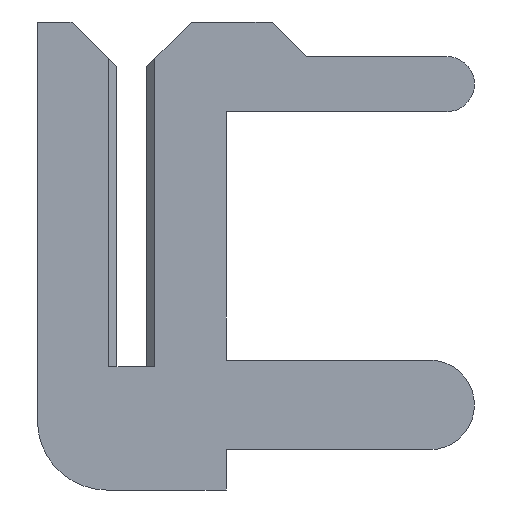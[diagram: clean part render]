
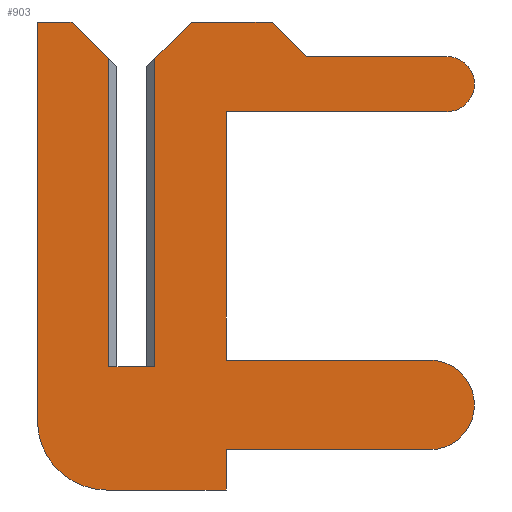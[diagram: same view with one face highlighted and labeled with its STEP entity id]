
A CAD part, left-side view. The second image highlights one B-rep face of the part: STEP entity #903.
In plain terms, the highlighted planar face has unit normal (-1, 0, 0).
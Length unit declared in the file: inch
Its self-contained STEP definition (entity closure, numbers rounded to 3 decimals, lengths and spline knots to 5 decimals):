
#18 = DIRECTION ( 'NONE',  ( 1., 0., 0. ) ) ;
#20 = ORIENTED_EDGE ( 'NONE', *, *, #310, .F. ) ;
#34 = CARTESIAN_POINT ( 'NONE',  ( -0.01, -0.01, 0. ) ) ;
#40 = DIRECTION ( 'NONE',  ( 0., -1., 0. ) ) ;
#46 = CARTESIAN_POINT ( 'NONE',  ( -0.01, 0.0065, 0.1305 ) ) ;
#50 = CIRCLE ( 'NONE', #1264, 0.0195 ) ;
#54 = CARTESIAN_POINT ( 'NONE',  ( -0.01, -0.1295, 0.003 ) ) ;
#63 = DIRECTION ( 'NONE',  ( 1., 0., 0. ) ) ;
#65 = ORIENTED_EDGE ( 'NONE', *, *, #385, .F. ) ;
#68 = LINE ( 'NONE', #1531, #400 ) ;
#90 = DIRECTION ( 'NONE',  ( 0., 0., 1. ) ) ;
#100 = LINE ( 'NONE', #1437, #1460 ) ;
#102 = DIRECTION ( 'NONE',  ( -1., 0., 0. ) ) ;
#108 = CARTESIAN_POINT ( 'NONE',  ( -0.01, -0.01, 0.15 ) ) ;
#116 = LINE ( 'NONE', #1648, #587 ) ;
#119 = EDGE_CURVE ( 'NONE', #751, #168, #161, .T. ) ;
#142 = ORIENTED_EDGE ( 'NONE', *, *, #1342, .F. ) ;
#144 = DIRECTION ( 'NONE',  ( 0., -1., 0. ) ) ;
#151 = DIRECTION ( 'NONE',  ( 0., 1., 0. ) ) ;
#161 = LINE ( 'NONE', #163, #275 ) ;
#163 = CARTESIAN_POINT ( 'NONE',  ( -0.01, -0.041, 0.003 ) ) ;
#168 = VERTEX_POINT ( 'NONE', #1359 ) ;
#171 = CARTESIAN_POINT ( 'NONE',  ( -0.01, -0.076, 0.135 ) ) ;
#186 = VECTOR ( 'NONE', #151, 39.37008 ) ;
#190 = ORIENTED_EDGE ( 'NONE', *, *, #600, .F. ) ;
#202 = EDGE_CURVE ( 'NONE', #232, #684, #116, .T. ) ;
#210 = LINE ( 'NONE', #171, #793 ) ;
#225 = EDGE_CURVE ( 'NONE', #646, #615, #210, .T. ) ;
#232 = VERTEX_POINT ( 'NONE', #857 ) ;
#237 = CARTESIAN_POINT ( 'NONE',  ( -0.01, -0.041, -0.0535 ) ) ;
#243 = LINE ( 'NONE', #108, #873 ) ;
#273 = CARTESIAN_POINT ( 'NONE',  ( -0.01, -0.041, -0.036 ) ) ;
#275 = VECTOR ( 'NONE', #322, 39.37008 ) ;
#282 = DIRECTION ( 'NONE',  ( 0., -1., 0. ) ) ;
#285 = AXIS2_PLACEMENT_3D ( 'NONE', #313, #295, #1224 ) ;
#289 = DIRECTION ( 'NONE',  ( 0., -1., 0. ) ) ;
#293 = CIRCLE ( 'NONE', #285, 0.012 ) ;
#295 = DIRECTION ( 'NONE',  ( 1., 0., 0. ) ) ;
#310 = EDGE_CURVE ( 'NONE', #804, #646, #1566, .T. ) ;
#313 = CARTESIAN_POINT ( 'NONE',  ( -0.01, -0.137, 0.123 ) ) ;
#322 = DIRECTION ( 'NONE',  ( 0., 0., -1. ) ) ;
#362 = ORIENTED_EDGE ( 'NONE', *, *, #409, .F. ) ;
#365 = EDGE_CURVE ( 'NONE', #1609, #751, #909, .T. ) ;
#378 = PLANE ( 'NONE',  #763 ) ;
#382 = VERTEX_POINT ( 'NONE', #826 ) ;
#385 = EDGE_CURVE ( 'NONE', #950, #1593, #1049, .T. ) ;
#394 = EDGE_CURVE ( 'NONE', #168, #704, #477, .T. ) ;
#400 = VECTOR ( 'NONE', #40, 39.37008 ) ;
#402 = EDGE_CURVE ( 'NONE', #864, #910, #649, .T. ) ;
#409 = EDGE_CURVE ( 'NONE', #1329, #1609, #293, .T. ) ;
#442 = CARTESIAN_POINT ( 'NONE',  ( -0.01, 0.011, -0.0235 ) ) ;
#447 = EDGE_LOOP ( 'NONE', ( #1201, #844, #142, #567, #190, #1583, #656, #65, #746, #1372, #1441, #817, #918, #871, #635, #362, #1209, #1106, #20 ) ) ;
#470 = EDGE_CURVE ( 'NONE', #615, #1329, #68, .T. ) ;
#477 = LINE ( 'NONE', #1346, #1645 ) ;
#515 = CARTESIAN_POINT ( 'NONE',  ( -0.01, -0.137, 0.135 ) ) ;
#527 = CARTESIAN_POINT ( 'NONE',  ( -0.01, 0.011, -0.0535 ) ) ;
#546 = VERTEX_POINT ( 'NONE', #34 ) ;
#560 = VECTOR ( 'NONE', #982, 39.37008 ) ;
#567 = ORIENTED_EDGE ( 'NONE', *, *, #202, .T. ) ;
#571 = CARTESIAN_POINT ( 'NONE',  ( -0.01, 0.026, 0.15 ) ) ;
#587 = VECTOR ( 'NONE', #850, 39.37008 ) ;
#600 = EDGE_CURVE ( 'NONE', #910, #684, #1675, .T. ) ;
#615 = VERTEX_POINT ( 'NONE', #1008 ) ;
#635 = ORIENTED_EDGE ( 'NONE', *, *, #365, .F. ) ;
#646 = VERTEX_POINT ( 'NONE', #1131 ) ;
#649 = LINE ( 'NONE', #571, #560 ) ;
#656 = ORIENTED_EDGE ( 'NONE', *, *, #707, .F. ) ;
#669 = AXIS2_PLACEMENT_3D ( 'NONE', #442, #18, #1483 ) ;
#684 = VERTEX_POINT ( 'NONE', #1391 ) ;
#686 = EDGE_CURVE ( 'NONE', #382, #950, #1277, .T. ) ;
#701 = CARTESIAN_POINT ( 'NONE',  ( -0.01, -0.137, 0.111 ) ) ;
#704 = VERTEX_POINT ( 'NONE', #54 ) ;
#707 = EDGE_CURVE ( 'NONE', #1593, #864, #1629, .T. ) ;
#718 = VECTOR ( 'NONE', #282, 39.37008 ) ;
#719 = DIRECTION ( 'NONE',  ( 0., -0.707, -0.707 ) ) ;
#733 = DIRECTION ( 'NONE',  ( 0., 1., 0. ) ) ;
#745 = CARTESIAN_POINT ( 'NONE',  ( -0.01, 0.041, 0.15 ) ) ;
#746 = ORIENTED_EDGE ( 'NONE', *, *, #686, .F. ) ;
#751 = VERTEX_POINT ( 'NONE', #1293 ) ;
#763 = AXIS2_PLACEMENT_3D ( 'NONE', #1172, #102, #1601 ) ;
#765 = CARTESIAN_POINT ( 'NONE',  ( -0.01, 0.026, 0.15 ) ) ;
#784 = EDGE_CURVE ( 'NONE', #1418, #382, #1396, .T. ) ;
#793 = VECTOR ( 'NONE', #1341, 39.37008 ) ;
#796 = EDGE_CURVE ( 'NONE', #704, #1394, #50, .T. ) ;
#802 = CARTESIAN_POINT ( 'NONE',  ( -0.01, 0.0065, 0. ) ) ;
#803 = VECTOR ( 'NONE', #733, 39.37008 ) ;
#804 = VERTEX_POINT ( 'NONE', #1282 ) ;
#817 = ORIENTED_EDGE ( 'NONE', *, *, #796, .F. ) ;
#826 = CARTESIAN_POINT ( 'NONE',  ( -0.01, -0.041, -0.0535 ) ) ;
#844 = ORIENTED_EDGE ( 'NONE', *, *, #1058, .T. ) ;
#850 = DIRECTION ( 'NONE',  ( 0., 0., 1. ) ) ;
#857 = CARTESIAN_POINT ( 'NONE',  ( -0.01, 0.01, 0. ) ) ;
#864 = VERTEX_POINT ( 'NONE', #912 ) ;
#871 = ORIENTED_EDGE ( 'NONE', *, *, #119, .F. ) ;
#873 = VECTOR ( 'NONE', #1442, 39.37008 ) ;
#895 = VECTOR ( 'NONE', #719, 39.37008 ) ;
#903 = ADVANCED_FACE ( 'NONE', ( #1230 ), #378, .T. ) ;
#909 = LINE ( 'NONE', #1644, #186 ) ;
#910 = VERTEX_POINT ( 'NONE', #765 ) ;
#912 = CARTESIAN_POINT ( 'NONE',  ( -0.01, 0.041, 0.15 ) ) ;
#918 = ORIENTED_EDGE ( 'NONE', *, *, #394, .F. ) ;
#927 = LINE ( 'NONE', #802, #718 ) ;
#932 = CARTESIAN_POINT ( 'NONE',  ( -0.01, -0.01, 0.134 ) ) ;
#950 = VERTEX_POINT ( 'NONE', #527 ) ;
#958 = EDGE_CURVE ( 'NONE', #1394, #1418, #100, .T. ) ;
#982 = DIRECTION ( 'NONE',  ( 0., -1., 0. ) ) ;
#1008 = CARTESIAN_POINT ( 'NONE',  ( -0.01, -0.076, 0.135 ) ) ;
#1020 = DIRECTION ( 'NONE',  ( 0., 0., -1. ) ) ;
#1049 = CIRCLE ( 'NONE', #669, 0.03 ) ;
#1056 = VECTOR ( 'NONE', #1489, 39.37008 ) ;
#1058 = EDGE_CURVE ( 'NONE', #1316, #546, #243, .T. ) ;
#1096 = CARTESIAN_POINT ( 'NONE',  ( -0.01, 0.041, -0.0235 ) ) ;
#1106 = ORIENTED_EDGE ( 'NONE', *, *, #225, .F. ) ;
#1131 = CARTESIAN_POINT ( 'NONE',  ( -0.01, -0.061, 0.15 ) ) ;
#1172 = CARTESIAN_POINT ( 'NONE',  ( -0.01, 0.011, -0.0235 ) ) ;
#1201 = ORIENTED_EDGE ( 'NONE', *, *, #1323, .F. ) ;
#1205 = VECTOR ( 'NONE', #144, 39.37008 ) ;
#1209 = ORIENTED_EDGE ( 'NONE', *, *, #470, .F. ) ;
#1224 = DIRECTION ( 'NONE',  ( 0., 0., 1. ) ) ;
#1230 = FACE_OUTER_BOUND ( 'NONE', #447, .T. ) ;
#1264 = AXIS2_PLACEMENT_3D ( 'NONE', #1427, #63, #90 ) ;
#1277 = LINE ( 'NONE', #1665, #803 ) ;
#1282 = CARTESIAN_POINT ( 'NONE',  ( -0.01, -0.026, 0.15 ) ) ;
#1293 = CARTESIAN_POINT ( 'NONE',  ( -0.01, -0.041, 0.111 ) ) ;
#1312 = CARTESIAN_POINT ( 'NONE',  ( -0.01, -0.0065, 0.1305 ) ) ;
#1316 = VERTEX_POINT ( 'NONE', #932 ) ;
#1323 = EDGE_CURVE ( 'NONE', #1316, #804, #1696, .T. ) ;
#1329 = VERTEX_POINT ( 'NONE', #515 ) ;
#1341 = DIRECTION ( 'NONE',  ( 0., -0.707, -0.707 ) ) ;
#1342 = EDGE_CURVE ( 'NONE', #232, #546, #927, .T. ) ;
#1346 = CARTESIAN_POINT ( 'NONE',  ( -0.01, -0.1295, 0.003 ) ) ;
#1359 = CARTESIAN_POINT ( 'NONE',  ( -0.01, -0.041, 0.003 ) ) ;
#1363 = CARTESIAN_POINT ( 'NONE',  ( -0.01, -0.026, 0.15 ) ) ;
#1372 = ORIENTED_EDGE ( 'NONE', *, *, #784, .F. ) ;
#1391 = CARTESIAN_POINT ( 'NONE',  ( -0.01, 0.01, 0.134 ) ) ;
#1394 = VERTEX_POINT ( 'NONE', #1608 ) ;
#1396 = LINE ( 'NONE', #237, #1699 ) ;
#1418 = VERTEX_POINT ( 'NONE', #273 ) ;
#1427 = CARTESIAN_POINT ( 'NONE',  ( -0.01, -0.1295, -0.0165 ) ) ;
#1437 = CARTESIAN_POINT ( 'NONE',  ( -0.01, -0.041, -0.036 ) ) ;
#1441 = ORIENTED_EDGE ( 'NONE', *, *, #958, .F. ) ;
#1442 = DIRECTION ( 'NONE',  ( 0., 0., -1. ) ) ;
#1460 = VECTOR ( 'NONE', #1725, 39.37008 ) ;
#1483 = DIRECTION ( 'NONE',  ( 0., 0., 1. ) ) ;
#1489 = DIRECTION ( 'NONE',  ( 0., -0.707, 0.707 ) ) ;
#1531 = CARTESIAN_POINT ( 'NONE',  ( -0.01, -0.137, 0.135 ) ) ;
#1558 = DIRECTION ( 'NONE',  ( 0., 0., 1. ) ) ;
#1566 = LINE ( 'NONE', #1363, #1205 ) ;
#1583 = ORIENTED_EDGE ( 'NONE', *, *, #402, .F. ) ;
#1592 = VECTOR ( 'NONE', #1558, 39.37008 ) ;
#1593 = VERTEX_POINT ( 'NONE', #1096 ) ;
#1601 = DIRECTION ( 'NONE',  ( 0., 0., 1. ) ) ;
#1608 = CARTESIAN_POINT ( 'NONE',  ( -0.01, -0.1295, -0.036 ) ) ;
#1609 = VERTEX_POINT ( 'NONE', #701 ) ;
#1629 = LINE ( 'NONE', #745, #1592 ) ;
#1644 = CARTESIAN_POINT ( 'NONE',  ( -0.01, -0.041, 0.111 ) ) ;
#1645 = VECTOR ( 'NONE', #289, 39.37008 ) ;
#1648 = CARTESIAN_POINT ( 'NONE',  ( -0.01, 0.01, -0.0235 ) ) ;
#1665 = CARTESIAN_POINT ( 'NONE',  ( -0.01, 0.011, -0.0535 ) ) ;
#1675 = LINE ( 'NONE', #46, #895 ) ;
#1696 = LINE ( 'NONE', #1312, #1056 ) ;
#1699 = VECTOR ( 'NONE', #1020, 39.37008 ) ;
#1725 = DIRECTION ( 'NONE',  ( 0., 1., 0. ) ) ;
